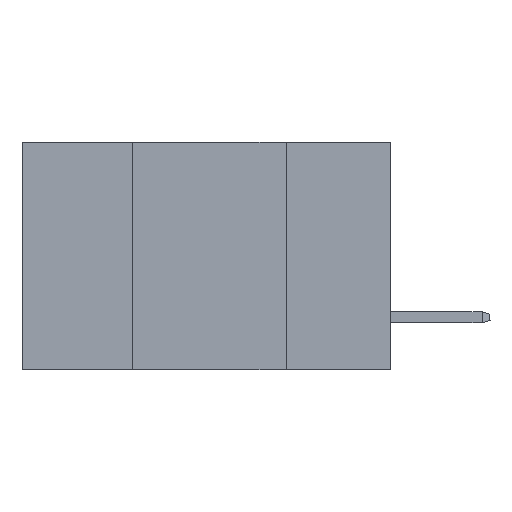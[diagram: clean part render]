
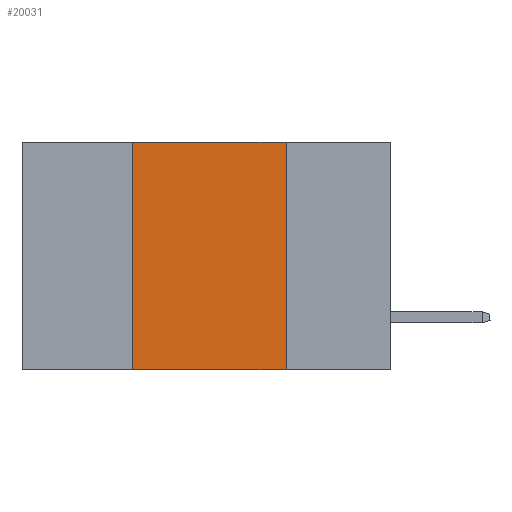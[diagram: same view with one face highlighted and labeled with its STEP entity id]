
A CAD part, left-side view. The second image highlights one B-rep face of the part: STEP entity #20031.
In plain terms, the highlighted planar face has unit normal (-1, 0, 0).
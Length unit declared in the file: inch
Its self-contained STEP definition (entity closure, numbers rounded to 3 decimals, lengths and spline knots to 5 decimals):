
#446 = VERTEX_POINT ( 'NONE', #31204 ) ;
#652 = DIRECTION ( 'NONE',  ( 1., 0., 0. ) ) ;
#832 = EDGE_CURVE ( 'NONE', #5022, #446, #12128, .T. ) ;
#901 = DIRECTION ( 'NONE',  ( 0., 0., -1. ) ) ;
#1464 = AXIS2_PLACEMENT_3D ( 'NONE', #17932, #652, #22661 ) ;
#3144 = LINE ( 'NONE', #21527, #18144 ) ;
#4102 = DIRECTION ( 'NONE',  ( 0., -1., 0. ) ) ;
#5022 = VERTEX_POINT ( 'NONE', #25694 ) ;
#5204 = VERTEX_POINT ( 'NONE', #31313 ) ;
#6005 = CARTESIAN_POINT ( 'NONE',  ( 0., 0.17, 0. ) ) ;
#6444 = VERTEX_POINT ( 'NONE', #28557 ) ;
#7325 = LINE ( 'NONE', #10330, #22309 ) ;
#10330 = CARTESIAN_POINT ( 'NONE',  ( 0., 0.42, 0. ) ) ;
#12076 = EDGE_CURVE ( 'NONE', #6444, #446, #13368, .T. ) ;
#12128 = LINE ( 'NONE', #6005, #15928 ) ;
#12953 = VECTOR ( 'NONE', #17527, 39.37008 ) ;
#13368 = LINE ( 'NONE', #15567, #12953 ) ;
#13586 = ORIENTED_EDGE ( 'NONE', *, *, #26300, .F. ) ;
#15467 = PLANE ( 'NONE',  #1464 ) ;
#15567 = CARTESIAN_POINT ( 'NONE',  ( 0., 0.6, -0.37 ) ) ;
#15928 = VECTOR ( 'NONE', #901, 39.37008 ) ;
#17258 = ORIENTED_EDGE ( 'NONE', *, *, #12076, .T. ) ;
#17527 = DIRECTION ( 'NONE',  ( 0., -1., 0. ) ) ;
#17724 = DIRECTION ( 'NONE',  ( 0., 0., 1. ) ) ;
#17932 = CARTESIAN_POINT ( 'NONE',  ( 0., 0.6, 0. ) ) ;
#17956 = EDGE_CURVE ( 'NONE', #6444, #5204, #7325, .T. ) ;
#18034 = EDGE_LOOP ( 'NONE', ( #27351, #13586, #28229, #17258 ) ) ;
#18144 = VECTOR ( 'NONE', #4102, 39.37008 ) ;
#20031 = ADVANCED_FACE ( 'NONE', ( #30133 ), #15467, .F. ) ;
#21527 = CARTESIAN_POINT ( 'NONE',  ( 0., 0.6, 0. ) ) ;
#22309 = VECTOR ( 'NONE', #17724, 39.37008 ) ;
#22661 = DIRECTION ( 'NONE',  ( 0., 0., -1. ) ) ;
#25694 = CARTESIAN_POINT ( 'NONE',  ( 0., 0.17, 0. ) ) ;
#26300 = EDGE_CURVE ( 'NONE', #5204, #5022, #3144, .T. ) ;
#27351 = ORIENTED_EDGE ( 'NONE', *, *, #832, .F. ) ;
#28229 = ORIENTED_EDGE ( 'NONE', *, *, #17956, .F. ) ;
#28557 = CARTESIAN_POINT ( 'NONE',  ( 0., 0.42, -0.37 ) ) ;
#30133 = FACE_OUTER_BOUND ( 'NONE', #18034, .T. ) ;
#31204 = CARTESIAN_POINT ( 'NONE',  ( 0., 0.17, -0.37 ) ) ;
#31313 = CARTESIAN_POINT ( 'NONE',  ( 0., 0.42, 0. ) ) ;
